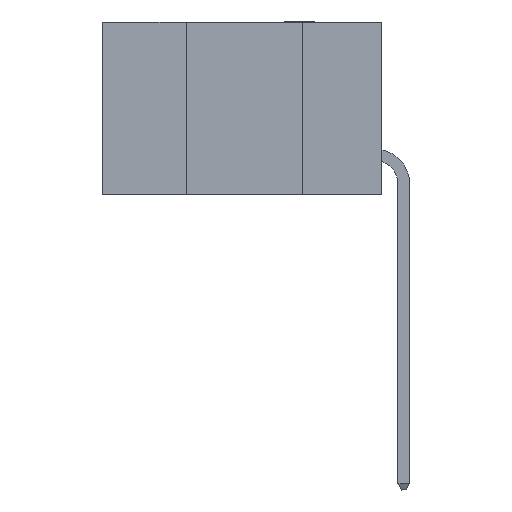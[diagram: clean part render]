
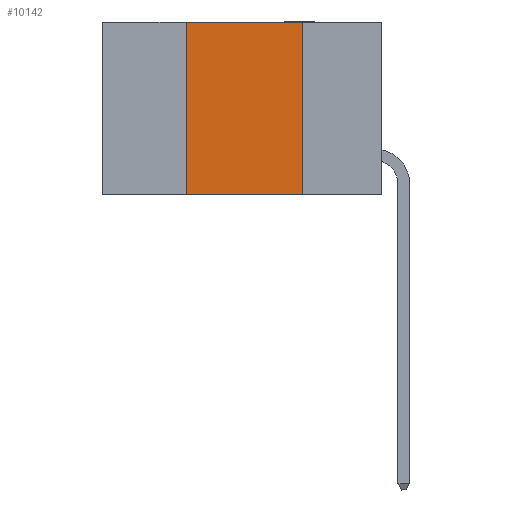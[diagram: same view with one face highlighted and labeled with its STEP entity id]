
A CAD part, left-side view. The second image highlights one B-rep face of the part: STEP entity #10142.
In plain terms, the highlighted planar face has unit normal (-1, 0, 0).
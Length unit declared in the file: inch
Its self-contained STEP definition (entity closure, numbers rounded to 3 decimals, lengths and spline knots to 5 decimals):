
#19 = VERTEX_POINT ( 'NONE', #10487 ) ;
#146 = VERTEX_POINT ( 'NONE', #253 ) ;
#253 = CARTESIAN_POINT ( 'NONE',  ( 0., 0.17, -0.37 ) ) ;
#350 = CARTESIAN_POINT ( 'NONE',  ( 0., 0.6, 0. ) ) ;
#1035 = VECTOR ( 'NONE', #17989, 39.37008 ) ;
#1242 = VECTOR ( 'NONE', #5185, 39.37008 ) ;
#1284 = ORIENTED_EDGE ( 'NONE', *, *, #12949, .F. ) ;
#1922 = ORIENTED_EDGE ( 'NONE', *, *, #11166, .T. ) ;
#2458 = VERTEX_POINT ( 'NONE', #7188 ) ;
#2928 = DIRECTION ( 'NONE',  ( 0., -1., 0. ) ) ;
#3205 = ORIENTED_EDGE ( 'NONE', *, *, #4825, .F. ) ;
#3305 = ORIENTED_EDGE ( 'NONE', *, *, #5829, .F. ) ;
#4081 = CARTESIAN_POINT ( 'NONE',  ( 0., 0.42, 0. ) ) ;
#4743 = LINE ( 'NONE', #14417, #1242 ) ;
#4825 = EDGE_CURVE ( 'NONE', #2458, #19, #11499, .T. ) ;
#5185 = DIRECTION ( 'NONE',  ( 0., 0., -1. ) ) ;
#5659 = DIRECTION ( 'NONE',  ( 0., 0., 1. ) ) ;
#5829 = EDGE_CURVE ( 'NONE', #19, #146, #4743, .T. ) ;
#6078 = FACE_OUTER_BOUND ( 'NONE', #12467, .T. ) ;
#6831 = CARTESIAN_POINT ( 'NONE',  ( 0., 0.6, 0. ) ) ;
#7188 = CARTESIAN_POINT ( 'NONE',  ( 0., 0.42, 0. ) ) ;
#9476 = CARTESIAN_POINT ( 'NONE',  ( 0., 0.6, -0.37 ) ) ;
#10142 = ADVANCED_FACE ( 'NONE', ( #6078 ), #18014, .F. ) ;
#10487 = CARTESIAN_POINT ( 'NONE',  ( 0., 0.17, 0. ) ) ;
#11166 = EDGE_CURVE ( 'NONE', #11971, #146, #17305, .T. ) ;
#11499 = LINE ( 'NONE', #6831, #1035 ) ;
#11971 = VERTEX_POINT ( 'NONE', #16594 ) ;
#12467 = EDGE_LOOP ( 'NONE', ( #3305, #3205, #1284, #1922 ) ) ;
#12949 = EDGE_CURVE ( 'NONE', #11971, #2458, #18192, .T. ) ;
#14417 = CARTESIAN_POINT ( 'NONE',  ( 0., 0.17, 0. ) ) ;
#14554 = VECTOR ( 'NONE', #2928, 39.37008 ) ;
#16594 = CARTESIAN_POINT ( 'NONE',  ( 0., 0.42, -0.37 ) ) ;
#16960 = VECTOR ( 'NONE', #5659, 39.37008 ) ;
#17305 = LINE ( 'NONE', #9476, #14554 ) ;
#17989 = DIRECTION ( 'NONE',  ( 0., -1., 0. ) ) ;
#18014 = PLANE ( 'NONE',  #19613 ) ;
#18192 = LINE ( 'NONE', #4081, #16960 ) ;
#19481 = DIRECTION ( 'NONE',  ( 0., 0., -1. ) ) ;
#19552 = DIRECTION ( 'NONE',  ( 1., 0., 0. ) ) ;
#19613 = AXIS2_PLACEMENT_3D ( 'NONE', #350, #19552, #19481 ) ;
